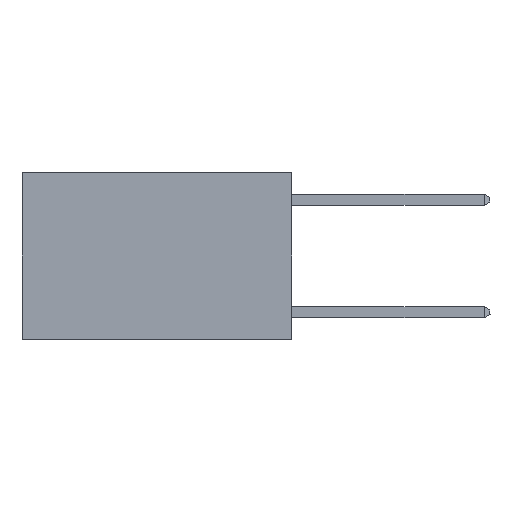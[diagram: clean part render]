
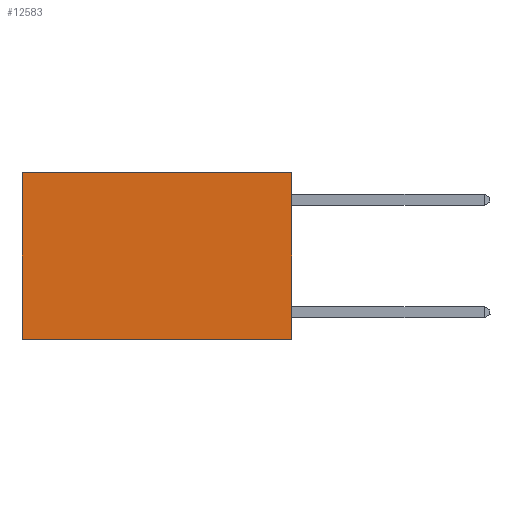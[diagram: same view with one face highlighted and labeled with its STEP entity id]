
A CAD part, left-side view. The second image highlights one B-rep face of the part: STEP entity #12583.
In plain terms, the highlighted planar face has unit normal (-1, 0, 0).
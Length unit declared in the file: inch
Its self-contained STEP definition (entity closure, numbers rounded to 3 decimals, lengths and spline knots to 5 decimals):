
#477 = CARTESIAN_POINT ( 'NONE',  ( 0.2625, 0., 0. ) ) ;
#514 = CARTESIAN_POINT ( 'NONE',  ( 0.2625, 0., 0. ) ) ;
#779 = CARTESIAN_POINT ( 'NONE',  ( 0.2625, 0., 0. ) ) ;
#1074 = VECTOR ( 'NONE', #12482, 39.37008 ) ;
#1495 = ORIENTED_EDGE ( 'NONE', *, *, #10005, .T. ) ;
#1623 = VERTEX_POINT ( 'NONE', #7570 ) ;
#2009 = AXIS2_PLACEMENT_3D ( 'NONE', #7714, #5792, #12465 ) ;
#2484 = LINE ( 'NONE', #514, #12443 ) ;
#2545 = CARTESIAN_POINT ( 'NONE',  ( 0.2625, 0., -0.37 ) ) ;
#2587 = VECTOR ( 'NONE', #9341, 39.37008 ) ;
#2992 = EDGE_LOOP ( 'NONE', ( #1495, #6692, #9390, #5567 ) ) ;
#3831 = EDGE_CURVE ( 'NONE', #11267, #1623, #2484, .T. ) ;
#4105 = CARTESIAN_POINT ( 'NONE',  ( 0.2625, 0.6, -0.37 ) ) ;
#4801 = VERTEX_POINT ( 'NONE', #4105 ) ;
#5567 = ORIENTED_EDGE ( 'NONE', *, *, #3831, .T. ) ;
#5640 = CARTESIAN_POINT ( 'NONE',  ( 0.2625, 0.6, 0. ) ) ;
#5792 = DIRECTION ( 'NONE',  ( 1., 0., 0. ) ) ;
#6385 = LINE ( 'NONE', #779, #1074 ) ;
#6692 = ORIENTED_EDGE ( 'NONE', *, *, #9909, .F. ) ;
#7570 = CARTESIAN_POINT ( 'NONE',  ( 0.2625, 0.6, 0. ) ) ;
#7714 = CARTESIAN_POINT ( 'NONE',  ( 0.2625, 0., 0. ) ) ;
#8244 = CARTESIAN_POINT ( 'NONE',  ( 0.2625, 0., -0.37 ) ) ;
#9341 = DIRECTION ( 'NONE',  ( 0., 1., 0. ) ) ;
#9390 = ORIENTED_EDGE ( 'NONE', *, *, #12043, .F. ) ;
#9909 = EDGE_CURVE ( 'NONE', #12382, #4801, #12527, .T. ) ;
#10005 = EDGE_CURVE ( 'NONE', #1623, #4801, #11384, .T. ) ;
#10389 = DIRECTION ( 'NONE',  ( 0., 1., 0. ) ) ;
#11267 = VERTEX_POINT ( 'NONE', #477 ) ;
#11316 = FACE_OUTER_BOUND ( 'NONE', #2992, .T. ) ;
#11384 = LINE ( 'NONE', #5640, #11664 ) ;
#11546 = PLANE ( 'NONE',  #2009 ) ;
#11664 = VECTOR ( 'NONE', #12326, 39.37008 ) ;
#12043 = EDGE_CURVE ( 'NONE', #11267, #12382, #6385, .T. ) ;
#12326 = DIRECTION ( 'NONE',  ( 0., 0., -1. ) ) ;
#12382 = VERTEX_POINT ( 'NONE', #8244 ) ;
#12443 = VECTOR ( 'NONE', #10389, 39.37008 ) ;
#12465 = DIRECTION ( 'NONE',  ( 0., 0., -1. ) ) ;
#12482 = DIRECTION ( 'NONE',  ( 0., 0., -1. ) ) ;
#12527 = LINE ( 'NONE', #2545, #2587 ) ;
#12583 = ADVANCED_FACE ( 'NONE', ( #11316 ), #11546, .F. ) ;
